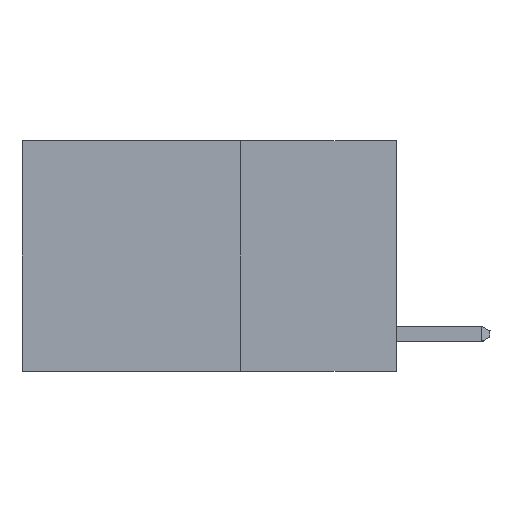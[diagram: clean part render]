
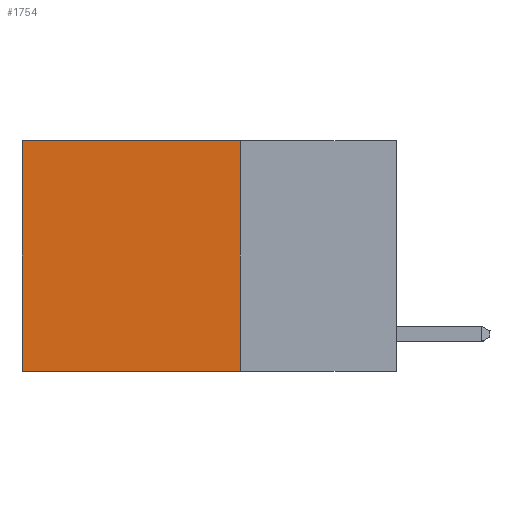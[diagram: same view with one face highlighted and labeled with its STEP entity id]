
A CAD part, left-side view. The second image highlights one B-rep face of the part: STEP entity #1754.
In plain terms, the highlighted planar face has unit normal (-1, 0, 0).
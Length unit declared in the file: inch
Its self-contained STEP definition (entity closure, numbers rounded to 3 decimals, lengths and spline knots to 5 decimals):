
#14 = CARTESIAN_POINT ( 'NONE',  ( 0.2625, 0.25, -0.37 ) ) ;
#242 = AXIS2_PLACEMENT_3D ( 'NONE', #5501, #5966, #5468 ) ;
#478 = CARTESIAN_POINT ( 'NONE',  ( 0.2625, 0.6, 0. ) ) ;
#545 = VECTOR ( 'NONE', #1728, 39.37008 ) ;
#574 = CARTESIAN_POINT ( 'NONE',  ( 0.2625, 0.6, -0.37 ) ) ;
#654 = EDGE_CURVE ( 'NONE', #6885, #3941, #6875, .T. ) ;
#756 = ORIENTED_EDGE ( 'NONE', *, *, #654, .T. ) ;
#980 = ORIENTED_EDGE ( 'NONE', *, *, #2672, .F. ) ;
#1039 = EDGE_CURVE ( 'NONE', #4257, #3941, #5533, .T. ) ;
#1174 = DIRECTION ( 'NONE',  ( 0., 0., -1. ) ) ;
#1728 = DIRECTION ( 'NONE',  ( 0., 1., 0. ) ) ;
#1729 = FACE_OUTER_BOUND ( 'NONE', #4618, .T. ) ;
#1754 = ADVANCED_FACE ( 'NONE', ( #1729 ), #4901, .F. ) ;
#1869 = DIRECTION ( 'NONE',  ( 0., 0., -1. ) ) ;
#2240 = CARTESIAN_POINT ( 'NONE',  ( 0.2625, 0.25, 0. ) ) ;
#2672 = EDGE_CURVE ( 'NONE', #4754, #4257, #7043, .T. ) ;
#3895 = ORIENTED_EDGE ( 'NONE', *, *, #3999, .T. ) ;
#3941 = VERTEX_POINT ( 'NONE', #574 ) ;
#3999 = EDGE_CURVE ( 'NONE', #4754, #6885, #7756, .T. ) ;
#4257 = VERTEX_POINT ( 'NONE', #5875 ) ;
#4379 = CARTESIAN_POINT ( 'NONE',  ( 0.2625, 0.25, 0. ) ) ;
#4618 = EDGE_LOOP ( 'NONE', ( #756, #6448, #980, #3895 ) ) ;
#4754 = VERTEX_POINT ( 'NONE', #4379 ) ;
#4901 = PLANE ( 'NONE',  #242 ) ;
#5468 = DIRECTION ( 'NONE',  ( 0., 0., -1. ) ) ;
#5501 = CARTESIAN_POINT ( 'NONE',  ( 0.2625, 0.25, 0. ) ) ;
#5533 = LINE ( 'NONE', #14, #545 ) ;
#5875 = CARTESIAN_POINT ( 'NONE',  ( 0.2625, 0.25, -0.37 ) ) ;
#5966 = DIRECTION ( 'NONE',  ( 1., 0., 0. ) ) ;
#6437 = CARTESIAN_POINT ( 'NONE',  ( 0.2625, 0.6, 0. ) ) ;
#6448 = ORIENTED_EDGE ( 'NONE', *, *, #1039, .F. ) ;
#6712 = VECTOR ( 'NONE', #1174, 39.37008 ) ;
#6875 = LINE ( 'NONE', #6437, #6712 ) ;
#6885 = VERTEX_POINT ( 'NONE', #478 ) ;
#6893 = VECTOR ( 'NONE', #1869, 39.37008 ) ;
#7043 = LINE ( 'NONE', #2240, #6893 ) ;
#7112 = DIRECTION ( 'NONE',  ( 0., 1., 0. ) ) ;
#7135 = CARTESIAN_POINT ( 'NONE',  ( 0.2625, 0.25, 0. ) ) ;
#7507 = VECTOR ( 'NONE', #7112, 39.37008 ) ;
#7756 = LINE ( 'NONE', #7135, #7507 ) ;
